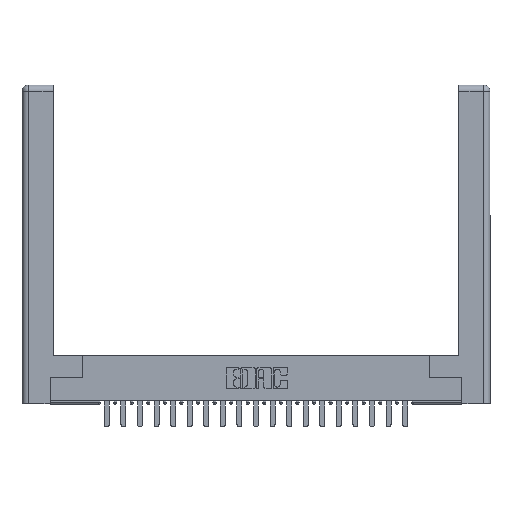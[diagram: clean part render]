
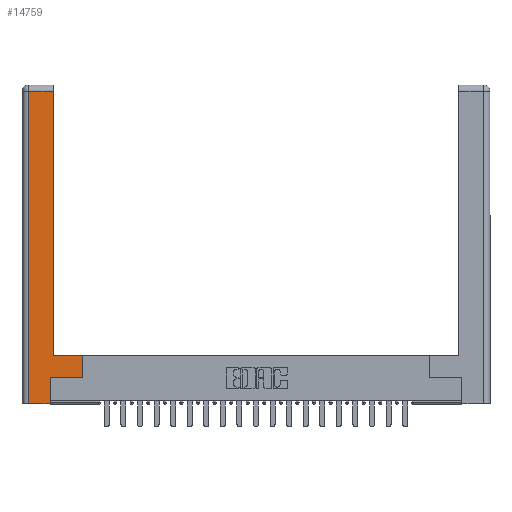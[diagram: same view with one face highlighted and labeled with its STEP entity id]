
A CAD part, top view. The second image highlights one B-rep face of the part: STEP entity #14759.
In plain terms, the highlighted planar face has unit normal (0, 0, 1).
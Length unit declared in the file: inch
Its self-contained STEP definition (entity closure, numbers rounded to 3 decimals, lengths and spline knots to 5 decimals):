
#613 = DIRECTION ( 'NONE',  ( 0., 0., -1. ) ) ;
#1206 = DIRECTION ( 'NONE',  ( -1., 0., 0. ) ) ;
#1240 = DIRECTION ( 'NONE',  ( -1., 0., 0. ) ) ;
#1292 = ORIENTED_EDGE ( 'NONE', *, *, #1782, .T. ) ;
#1782 = EDGE_CURVE ( 'NONE', #5493, #19303, #19211, .T. ) ;
#1809 = VERTEX_POINT ( 'NONE', #19873 ) ;
#2359 = DIRECTION ( 'NONE',  ( 0., 1., 0. ) ) ;
#2978 = CARTESIAN_POINT ( 'NONE',  ( 0.565, 0.45, 0. ) ) ;
#3065 = CARTESIAN_POINT ( 'NONE',  ( 0.0615, 0., 0. ) ) ;
#3813 = CARTESIAN_POINT ( 'NONE',  ( 0.565, 0.245, 0. ) ) ;
#3878 = LINE ( 'NONE', #4101, #14806 ) ;
#4101 = CARTESIAN_POINT ( 'NONE',  ( 0.565, 0.45, 0. ) ) ;
#5327 = VERTEX_POINT ( 'NONE', #19006 ) ;
#5493 = VERTEX_POINT ( 'NONE', #7181 ) ;
#5805 = CARTESIAN_POINT ( 'NONE',  ( 0., 0., 0. ) ) ;
#6390 = CARTESIAN_POINT ( 'NONE',  ( 0.295, 0.45, 0. ) ) ;
#7160 = CARTESIAN_POINT ( 'NONE',  ( 0.565, 0.245, 0. ) ) ;
#7181 = CARTESIAN_POINT ( 'NONE',  ( 0.0615, 2.94, 0. ) ) ;
#7292 = LINE ( 'NONE', #16050, #13534 ) ;
#7654 = ORIENTED_EDGE ( 'NONE', *, *, #14113, .T. ) ;
#8221 = VECTOR ( 'NONE', #18541, 39.37008 ) ;
#8255 = ORIENTED_EDGE ( 'NONE', *, *, #22386, .T. ) ;
#8942 = EDGE_LOOP ( 'NONE', ( #21399, #8255, #1292, #7654, #14258, #13334, #22608, #20637 ) ) ;
#9223 = VERTEX_POINT ( 'NONE', #3813 ) ;
#9478 = DIRECTION ( 'NONE',  ( -1., 0., 0. ) ) ;
#10760 = EDGE_CURVE ( 'NONE', #18155, #5327, #15719, .T. ) ;
#10921 = DIRECTION ( 'NONE',  ( 1., 0., 0. ) ) ;
#11357 = CARTESIAN_POINT ( 'NONE',  ( 0.265, 0.245, 0. ) ) ;
#12417 = EDGE_CURVE ( 'NONE', #16870, #21896, #16671, .T. ) ;
#12636 = EDGE_CURVE ( 'NONE', #5327, #1809, #7292, .T. ) ;
#13334 = ORIENTED_EDGE ( 'NONE', *, *, #21714, .T. ) ;
#13534 = VECTOR ( 'NONE', #17689, 39.37008 ) ;
#13694 = DIRECTION ( 'NONE',  ( 0., -1., 0. ) ) ;
#14113 = EDGE_CURVE ( 'NONE', #19303, #16870, #14573, .T. ) ;
#14258 = ORIENTED_EDGE ( 'NONE', *, *, #12417, .T. ) ;
#14383 = DIRECTION ( 'NONE',  ( 1., 0., 0. ) ) ;
#14573 = LINE ( 'NONE', #21508, #19151 ) ;
#14759 = ADVANCED_FACE ( 'NONE', ( #15247 ), #21957, .F. ) ;
#14806 = VECTOR ( 'NONE', #2359, 39.37008 ) ;
#14818 = VECTOR ( 'NONE', #1240, 39.37008 ) ;
#15066 = AXIS2_PLACEMENT_3D ( 'NONE', #5805, #613, #9478 ) ;
#15247 = FACE_OUTER_BOUND ( 'NONE', #8942, .T. ) ;
#15719 = LINE ( 'NONE', #6390, #21036 ) ;
#15916 = VECTOR ( 'NONE', #14383, 39.37008 ) ;
#16050 = CARTESIAN_POINT ( 'NONE',  ( 0.295, 3., 0. ) ) ;
#16671 = LINE ( 'NONE', #11357, #8221 ) ;
#16870 = VERTEX_POINT ( 'NONE', #22573 ) ;
#17163 = LINE ( 'NONE', #17394, #14818 ) ;
#17394 = CARTESIAN_POINT ( 'NONE',  ( 0.0615, 2.94, 0. ) ) ;
#17689 = DIRECTION ( 'NONE',  ( 0., 1., 0. ) ) ;
#17796 = LINE ( 'NONE', #7160, #15916 ) ;
#18155 = VERTEX_POINT ( 'NONE', #2978 ) ;
#18541 = DIRECTION ( 'NONE',  ( 0., 1., 0. ) ) ;
#19006 = CARTESIAN_POINT ( 'NONE',  ( 0.295, 0.45, 0. ) ) ;
#19151 = VECTOR ( 'NONE', #10921, 39.37008 ) ;
#19211 = LINE ( 'NONE', #3065, #22304 ) ;
#19303 = VERTEX_POINT ( 'NONE', #22225 ) ;
#19873 = CARTESIAN_POINT ( 'NONE',  ( 0.295, 2.94, 0. ) ) ;
#20063 = EDGE_CURVE ( 'NONE', #9223, #18155, #3878, .T. ) ;
#20260 = CARTESIAN_POINT ( 'NONE',  ( 0.265, 0.245, 0. ) ) ;
#20637 = ORIENTED_EDGE ( 'NONE', *, *, #10760, .T. ) ;
#21036 = VECTOR ( 'NONE', #1206, 39.37008 ) ;
#21399 = ORIENTED_EDGE ( 'NONE', *, *, #12636, .T. ) ;
#21508 = CARTESIAN_POINT ( 'NONE',  ( 0.265, 0., 0. ) ) ;
#21714 = EDGE_CURVE ( 'NONE', #21896, #9223, #17796, .T. ) ;
#21896 = VERTEX_POINT ( 'NONE', #20260 ) ;
#21957 = PLANE ( 'NONE',  #15066 ) ;
#22225 = CARTESIAN_POINT ( 'NONE',  ( 0.0615, 0., 0. ) ) ;
#22304 = VECTOR ( 'NONE', #13694, 39.37008 ) ;
#22386 = EDGE_CURVE ( 'NONE', #1809, #5493, #17163, .T. ) ;
#22573 = CARTESIAN_POINT ( 'NONE',  ( 0.265, 0., 0. ) ) ;
#22608 = ORIENTED_EDGE ( 'NONE', *, *, #20063, .T. ) ;
